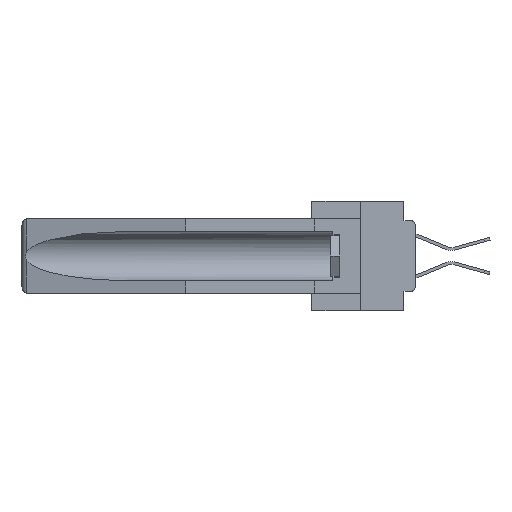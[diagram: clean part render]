
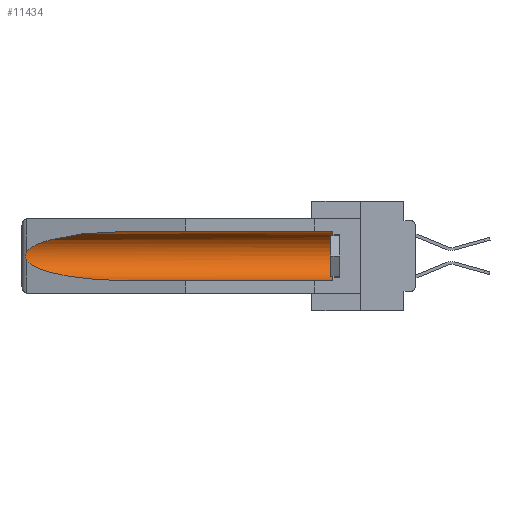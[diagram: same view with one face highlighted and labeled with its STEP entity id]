
A CAD part, left-side view. The second image highlights one B-rep face of the part: STEP entity #11434.
In plain terms, the highlighted cylindrical face has radius 2.857 mm (diameter 5.715 mm), a partial arc.
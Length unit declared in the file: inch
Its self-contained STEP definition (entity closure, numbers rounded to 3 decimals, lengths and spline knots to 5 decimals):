
#904 = ORIENTED_EDGE ( 'NONE', *, *, #14621, .F. ) ;
#1380 = CARTESIAN_POINT ( 'NONE',  ( 0.25451, 1.48313, -0.09465 ) ) ;
#1409 = VERTEX_POINT ( 'NONE', #8054 ) ;
#1609 = CARTESIAN_POINT ( 'NONE',  ( 0.155, 0.126, -0.059 ) ) ;
#1637 =( BOUNDED_CURVE ( )  B_SPLINE_CURVE ( 3, ( #21242, #14343, #14545, #25654 ),
 .UNSPECIFIED., .F., .T. ) 
 B_SPLINE_CURVE_WITH_KNOTS ( ( 4, 4 ),
 ( 0.1948, 1.5708 ),
 .UNSPECIFIED. ) 
 CURVE ( )  GEOMETRIC_REPRESENTATION_ITEM ( )  RATIONAL_B_SPLINE_CURVE ( ( 1., 0.848, 0.848, 1. ) ) 
 REPRESENTATION_ITEM ( '' )  );
#3124 = ORIENTED_EDGE ( 'NONE', *, *, #6715, .T. ) ;
#3310 = VERTEX_POINT ( 'NONE', #22425 ) ;
#3520 = CARTESIAN_POINT ( 'NONE',  ( 0.155, -0.30754, -0.1715 ) ) ;
#4119 = ORIENTED_EDGE ( 'NONE', *, *, #22640, .T. ) ;
#4686 = EDGE_CURVE ( 'NONE', #8876, #21881, #8782, .T. ) ;
#5223 = DIRECTION ( 'NONE',  ( 0., -1., 0. ) ) ;
#5249 = EDGE_CURVE ( 'NONE', #19756, #8876, #28487, .T. ) ;
#6427 = CARTESIAN_POINT ( 'NONE',  ( 0.155, 0.126, -0.284 ) ) ;
#6715 = EDGE_CURVE ( 'NONE', #21881, #8287, #29076, .T. ) ;
#6730 = AXIS2_PLACEMENT_3D ( 'NONE', #3520, #26091, #10402 ) ;
#7112 = CARTESIAN_POINT ( 'NONE',  ( 0.26597, 1.5296, -0.19026 ) ) ;
#7404 = CARTESIAN_POINT ( 'NONE',  ( 0.26654, 1.53092, -0.15636 ) ) ;
#8054 = CARTESIAN_POINT ( 'NONE',  ( 0.155, 1.07973, -0.284 ) ) ;
#8287 = VERTEX_POINT ( 'NONE', #19529 ) ;
#8782 = LINE ( 'NONE', #21403, #12682 ) ;
#8876 = VERTEX_POINT ( 'NONE', #1609 ) ;
#9363 = CARTESIAN_POINT ( 'NONE',  ( 0.2675, 1.53308, -0.17534 ) ) ;
#9725 = CARTESIAN_POINT ( 'NONE',  ( 0.155, -0.30754, -0.284 ) ) ;
#10016 = DIRECTION ( 'NONE',  ( 0., 1., 0. ) ) ;
#10402 = DIRECTION ( 'NONE',  ( 0., 0., 1. ) ) ;
#10851 = B_SPLINE_CURVE_WITH_KNOTS ( 'NONE', 3,
 ( #16377, #18419, #7404, #25327, #25229, #9363, #18513, #22973, #7112, #23166 ),
 .UNSPECIFIED., .F., .F.,
 ( 4, 2, 2, 2, 4 ),
 ( 0., 0.00029, 0.00058, 0.00087, 0.00117 ),
 .UNSPECIFIED. ) ;
#11038 = ORIENTED_EDGE ( 'NONE', *, *, #23122, .T. ) ;
#11434 = ADVANCED_FACE ( 'NONE', ( #26687 ), #20713, .F. ) ;
#12218 = CARTESIAN_POINT ( 'NONE',  ( 0.155, 0.126, -0.1715 ) ) ;
#12682 = VECTOR ( 'NONE', #28000, 39.37008 ) ;
#12776 = LINE ( 'NONE', #9725, #23334 ) ;
#13316 = CARTESIAN_POINT ( 'NONE',  ( 0.21114, 1.30732, -0.059 ) ) ;
#14343 = CARTESIAN_POINT ( 'NONE',  ( 0.25451, 1.48313, -0.24835 ) ) ;
#14545 = CARTESIAN_POINT ( 'NONE',  ( 0.21114, 1.30732, -0.284 ) ) ;
#14621 = EDGE_CURVE ( 'NONE', #19756, #1409, #12776, .T. ) ;
#15574 = CARTESIAN_POINT ( 'NONE',  ( 0.26537, 1.52718, -0.14972 ) ) ;
#16377 = CARTESIAN_POINT ( 'NONE',  ( 0.26537, 1.52718, -0.14972 ) ) ;
#17650 = EDGE_LOOP ( 'NONE', ( #3124, #11038, #4119, #904, #18047, #23452 ) ) ;
#18047 = ORIENTED_EDGE ( 'NONE', *, *, #5249, .T. ) ;
#18419 = CARTESIAN_POINT ( 'NONE',  ( 0.26597, 1.52961, -0.15275 ) ) ;
#18513 = CARTESIAN_POINT ( 'NONE',  ( 0.2673, 1.53269, -0.17917 ) ) ;
#19529 = CARTESIAN_POINT ( 'NONE',  ( 0.26537, 1.52718, -0.14972 ) ) ;
#19756 = VERTEX_POINT ( 'NONE', #6427 ) ;
#20441 = AXIS2_PLACEMENT_3D ( 'NONE', #12218, #5223, #27879 ) ;
#20713 = CYLINDRICAL_SURFACE ( 'NONE', #6730, 0.1125 ) ;
#21242 = CARTESIAN_POINT ( 'NONE',  ( 0.26537, 1.52718, -0.19328 ) ) ;
#21403 = CARTESIAN_POINT ( 'NONE',  ( 0.155, -0.30754, -0.059 ) ) ;
#21881 = VERTEX_POINT ( 'NONE', #27030 ) ;
#22425 = CARTESIAN_POINT ( 'NONE',  ( 0.26537, 1.52718, -0.19328 ) ) ;
#22640 = EDGE_CURVE ( 'NONE', #3310, #1409, #1637, .T. ) ;
#22973 = CARTESIAN_POINT ( 'NONE',  ( 0.26655, 1.53094, -0.18657 ) ) ;
#23122 = EDGE_CURVE ( 'NONE', #8287, #3310, #10851, .T. ) ;
#23166 = CARTESIAN_POINT ( 'NONE',  ( 0.26537, 1.52718, -0.19328 ) ) ;
#23334 = VECTOR ( 'NONE', #10016, 39.37008 ) ;
#23452 = ORIENTED_EDGE ( 'NONE', *, *, #4686, .T. ) ;
#25229 = CARTESIAN_POINT ( 'NONE',  ( 0.2675, 1.53308, -0.16763 ) ) ;
#25327 = CARTESIAN_POINT ( 'NONE',  ( 0.2673, 1.5327, -0.16383 ) ) ;
#25654 = CARTESIAN_POINT ( 'NONE',  ( 0.155, 1.07973, -0.284 ) ) ;
#26091 = DIRECTION ( 'NONE',  ( 0., 1., 0. ) ) ;
#26687 = FACE_OUTER_BOUND ( 'NONE', #17650, .T. ) ;
#26802 = CARTESIAN_POINT ( 'NONE',  ( 0.155, 1.07973, -0.059 ) ) ;
#27030 = CARTESIAN_POINT ( 'NONE',  ( 0.155, 1.07973, -0.059 ) ) ;
#27879 = DIRECTION ( 'NONE',  ( 0., 0., 1. ) ) ;
#28000 = DIRECTION ( 'NONE',  ( 0., 1., 0. ) ) ;
#28487 = CIRCLE ( 'NONE', #20441, 0.1125 ) ;
#29076 =( BOUNDED_CURVE ( )  B_SPLINE_CURVE ( 3, ( #26802, #13316, #1380, #15574 ),
 .UNSPECIFIED., .F., .F. ) 
 B_SPLINE_CURVE_WITH_KNOTS ( ( 4, 4 ),
 ( 4.71239, 6.08839 ),
 .UNSPECIFIED. ) 
 CURVE ( )  GEOMETRIC_REPRESENTATION_ITEM ( )  RATIONAL_B_SPLINE_CURVE ( ( 1., 0.848, 0.848, 1. ) ) 
 REPRESENTATION_ITEM ( '' )  );
